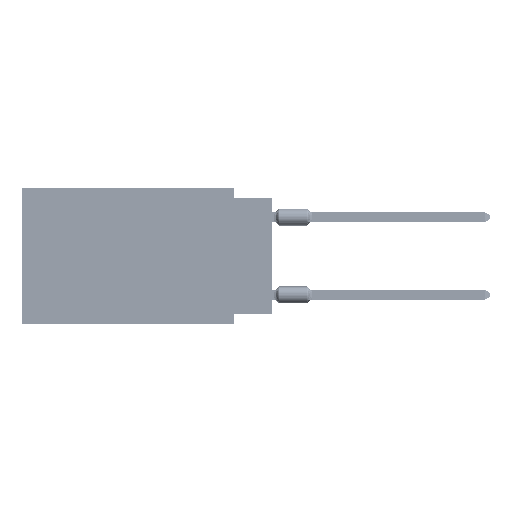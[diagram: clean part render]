
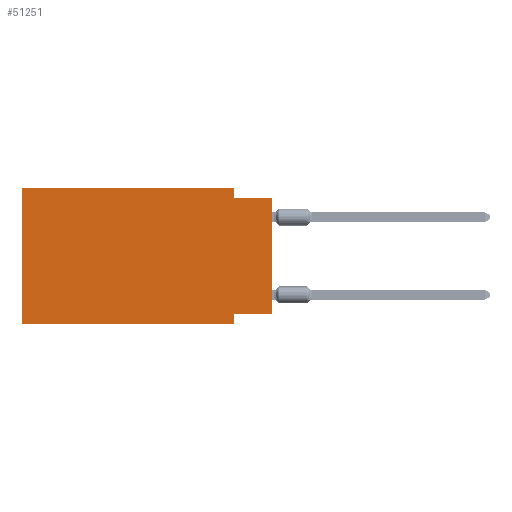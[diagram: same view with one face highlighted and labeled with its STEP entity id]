
A CAD part, left-side view. The second image highlights one B-rep face of the part: STEP entity #51251.
In plain terms, the highlighted planar face has unit normal (-1, 0, 0).
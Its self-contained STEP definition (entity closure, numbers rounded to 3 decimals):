
#40 = VECTOR ( 'NONE', #94445, 1000. ) ;
#2317 = CARTESIAN_POINT ( 'NONE',  ( 0., 0., -8.255 ) ) ;
#2964 = CARTESIAN_POINT ( 'NONE',  ( 0., 2.54, -8.89 ) ) ;
#5032 = EDGE_CURVE ( 'NONE', #74998, #59410, #57860, .T. ) ;
#5362 = FACE_OUTER_BOUND ( 'NONE', #46672, .T. ) ;
#6384 = DIRECTION ( 'NONE',  ( 1., 0., 0. ) ) ;
#6731 = AXIS2_PLACEMENT_3D ( 'NONE', #76804, #6384, #60376 ) ;
#7615 = LINE ( 'NONE', #15327, #32124 ) ;
#9618 = ORIENTED_EDGE ( 'NONE', *, *, #69736, .F. ) ;
#11121 = EDGE_CURVE ( 'NONE', #17582, #83670, #7615, .T. ) ;
#11835 = LINE ( 'NONE', #42180, #62666 ) ;
#15327 = CARTESIAN_POINT ( 'NONE',  ( 0., 0., 0. ) ) ;
#17582 = VERTEX_POINT ( 'NONE', #2317 ) ;
#24510 = LINE ( 'NONE', #63081, #40 ) ;
#24765 = DIRECTION ( 'NONE',  ( 0., 0., -1. ) ) ;
#27001 = DIRECTION ( 'NONE',  ( 0., -1., 0. ) ) ;
#30173 = LINE ( 'NONE', #75924, #50846 ) ;
#30659 = DIRECTION ( 'NONE',  ( 0., 0., 1. ) ) ;
#32052 = ORIENTED_EDGE ( 'NONE', *, *, #90229, .F. ) ;
#32124 = VECTOR ( 'NONE', #55396, 1000. ) ;
#32993 = LINE ( 'NONE', #33496, #37091 ) ;
#33496 = CARTESIAN_POINT ( 'NONE',  ( 0., 2.54, 0. ) ) ;
#33634 = EDGE_CURVE ( 'NONE', #17582, #51872, #11835, .T. ) ;
#35296 = VERTEX_POINT ( 'NONE', #84653 ) ;
#37091 = VECTOR ( 'NONE', #24765, 1000. ) ;
#38369 = ORIENTED_EDGE ( 'NONE', *, *, #11121, .T. ) ;
#42180 = CARTESIAN_POINT ( 'NONE',  ( 0., 0., -8.255 ) ) ;
#46672 = EDGE_LOOP ( 'NONE', ( #38369, #88657, #74066, #32052, #9618, #81660, #54764, #92260 ) ) ;
#50846 = VECTOR ( 'NONE', #53281, 1000. ) ;
#51251 = ADVANCED_FACE ( 'NONE', ( #5362 ), #68072, .F. ) ;
#51872 = VERTEX_POINT ( 'NONE', #96200 ) ;
#53258 = LINE ( 'NONE', #101077, #87280 ) ;
#53281 = DIRECTION ( 'NONE',  ( 0., -1., 0. ) ) ;
#54764 = ORIENTED_EDGE ( 'NONE', *, *, #69524, .F. ) ;
#55225 = VERTEX_POINT ( 'NONE', #67074 ) ;
#55396 = DIRECTION ( 'NONE',  ( 0., 0., 1. ) ) ;
#56020 = VECTOR ( 'NONE', #73406, 1000. ) ;
#57860 = LINE ( 'NONE', #89221, #67394 ) ;
#58031 = CARTESIAN_POINT ( 'NONE',  ( 0., 0., -0.635 ) ) ;
#59410 = VERTEX_POINT ( 'NONE', #85163 ) ;
#60376 = DIRECTION ( 'NONE',  ( 0., 0., -1. ) ) ;
#60935 = VERTEX_POINT ( 'NONE', #65181 ) ;
#62666 = VECTOR ( 'NONE', #73536, 1000. ) ;
#63081 = CARTESIAN_POINT ( 'NONE',  ( 0., 0., -0.635 ) ) ;
#65181 = CARTESIAN_POINT ( 'NONE',  ( 0., 2.54, -0.635 ) ) ;
#67074 = CARTESIAN_POINT ( 'NONE',  ( 0., 16.383, 0. ) ) ;
#67394 = VECTOR ( 'NONE', #27001, 1000. ) ;
#68072 = PLANE ( 'NONE',  #6731 ) ;
#69524 = EDGE_CURVE ( 'NONE', #51872, #59410, #73908, .T. ) ;
#69736 = EDGE_CURVE ( 'NONE', #74998, #55225, #53258, .T. ) ;
#73406 = DIRECTION ( 'NONE',  ( 0., 0., -1. ) ) ;
#73536 = DIRECTION ( 'NONE',  ( 0., 1., 0. ) ) ;
#73908 = LINE ( 'NONE', #2964, #56020 ) ;
#74066 = ORIENTED_EDGE ( 'NONE', *, *, #75353, .F. ) ;
#74998 = VERTEX_POINT ( 'NONE', #95948 ) ;
#75353 = EDGE_CURVE ( 'NONE', #35296, #60935, #32993, .T. ) ;
#75924 = CARTESIAN_POINT ( 'NONE',  ( 0., 16.383, 0. ) ) ;
#76804 = CARTESIAN_POINT ( 'NONE',  ( 0., 16.383, 0. ) ) ;
#81660 = ORIENTED_EDGE ( 'NONE', *, *, #5032, .T. ) ;
#83670 = VERTEX_POINT ( 'NONE', #58031 ) ;
#84653 = CARTESIAN_POINT ( 'NONE',  ( 0., 2.54, 0. ) ) ;
#85163 = CARTESIAN_POINT ( 'NONE',  ( 0., 2.54, -8.89 ) ) ;
#87280 = VECTOR ( 'NONE', #30659, 1000. ) ;
#88657 = ORIENTED_EDGE ( 'NONE', *, *, #91730, .F. ) ;
#89221 = CARTESIAN_POINT ( 'NONE',  ( 0., 16.383, -8.89 ) ) ;
#90229 = EDGE_CURVE ( 'NONE', #55225, #35296, #30173, .T. ) ;
#91730 = EDGE_CURVE ( 'NONE', #60935, #83670, #24510, .T. ) ;
#92260 = ORIENTED_EDGE ( 'NONE', *, *, #33634, .F. ) ;
#94445 = DIRECTION ( 'NONE',  ( 0., -1., 0. ) ) ;
#95948 = CARTESIAN_POINT ( 'NONE',  ( 0., 16.383, -8.89 ) ) ;
#96200 = CARTESIAN_POINT ( 'NONE',  ( 0., 2.54, -8.255 ) ) ;
#101077 = CARTESIAN_POINT ( 'NONE',  ( 0., 16.383, 0. ) ) ;
